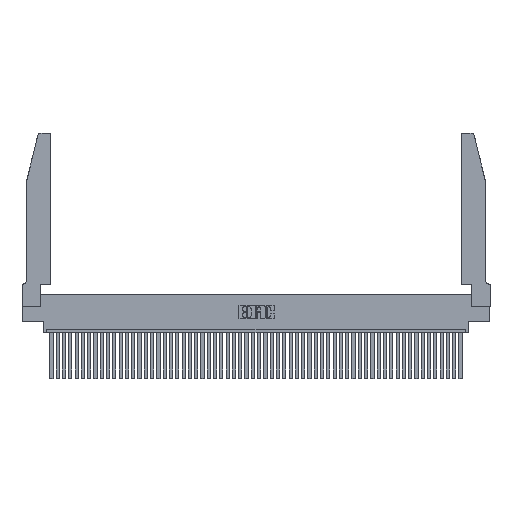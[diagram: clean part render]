
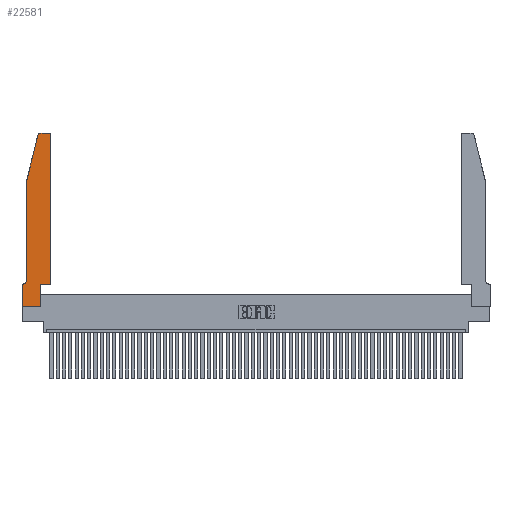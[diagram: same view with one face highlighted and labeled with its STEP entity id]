
A CAD part, top view. The second image highlights one B-rep face of the part: STEP entity #22581.
In plain terms, the highlighted planar face has unit normal (0, 0, 1).
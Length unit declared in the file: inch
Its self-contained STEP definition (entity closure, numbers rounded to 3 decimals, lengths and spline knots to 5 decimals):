
#289 = EDGE_CURVE ( 'NONE', #35568, #41114, #4312, .T. ) ;
#635 = ORIENTED_EDGE ( 'NONE', *, *, #289, .T. ) ;
#738 = AXIS2_PLACEMENT_3D ( 'NONE', #3399, #35102, #23356 ) ;
#847 = VERTEX_POINT ( 'NONE', #31609 ) ;
#1453 = VECTOR ( 'NONE', #14521, 39.37008 ) ;
#2069 = DIRECTION ( 'NONE',  ( -0.239, -0.971, 0. ) ) ;
#2330 = CARTESIAN_POINT ( 'NONE',  ( 0., 0., 0.37 ) ) ;
#2375 = LINE ( 'NONE', #38736, #33975 ) ;
#2720 = CARTESIAN_POINT ( 'NONE',  ( 0.4505, 0.35, 0.37 ) ) ;
#2827 = ORIENTED_EDGE ( 'NONE', *, *, #40851, .T. ) ;
#3399 = CARTESIAN_POINT ( 'NONE',  ( 0.0055, 0.42, 0.37 ) ) ;
#3774 = VERTEX_POINT ( 'NONE', #2330 ) ;
#4251 = CARTESIAN_POINT ( 'NONE',  ( 0.0055, 0.35, 0.37 ) ) ;
#4275 = DIRECTION ( 'NONE',  ( -1., 0., 0. ) ) ;
#4312 = LINE ( 'NONE', #29773, #12376 ) ;
#4354 = CARTESIAN_POINT ( 'NONE',  ( 0.0755, 2., 0.37 ) ) ;
#6153 = DIRECTION ( 'NONE',  ( 0., -1., 0. ) ) ;
#6306 = CARTESIAN_POINT ( 'NONE',  ( 0.0755, 0.35, 0.37 ) ) ;
#6374 = DIRECTION ( 'NONE',  ( 1., 0., 0. ) ) ;
#6639 = DIRECTION ( 'NONE',  ( 0., 0., 1. ) ) ;
#7251 = DIRECTION ( 'NONE',  ( 1., 0., 0. ) ) ;
#8568 = ORIENTED_EDGE ( 'NONE', *, *, #30644, .T. ) ;
#9077 = LINE ( 'NONE', #23287, #9700 ) ;
#9700 = VECTOR ( 'NONE', #30693, 39.37008 ) ;
#9938 = CARTESIAN_POINT ( 'NONE',  ( 0.4505, 0.35, 0.37 ) ) ;
#10612 = PLANE ( 'NONE',  #38066 ) ;
#11401 = VERTEX_POINT ( 'NONE', #32820 ) ;
#11506 = EDGE_CURVE ( 'NONE', #3774, #25291, #43487, .T. ) ;
#12145 = VERTEX_POINT ( 'NONE', #9938 ) ;
#12376 = VECTOR ( 'NONE', #2069, 39.37008 ) ;
#12937 = AXIS2_PLACEMENT_3D ( 'NONE', #29417, #33943, #45576 ) ;
#13068 = EDGE_CURVE ( 'NONE', #48024, #13459, #20467, .T. ) ;
#13267 = CARTESIAN_POINT ( 'NONE',  ( 0.284, 2.75, 0.37 ) ) ;
#13459 = VERTEX_POINT ( 'NONE', #18127 ) ;
#14521 = DIRECTION ( 'NONE',  ( 0., 1., 0. ) ) ;
#14974 = CARTESIAN_POINT ( 'NONE',  ( 0., 0., 0.37 ) ) ;
#15345 = CARTESIAN_POINT ( 'NONE',  ( 0.2865, 0., 0.37 ) ) ;
#15667 = EDGE_CURVE ( 'NONE', #15916, #847, #38754, .T. ) ;
#15916 = VERTEX_POINT ( 'NONE', #4251 ) ;
#16276 = CIRCLE ( 'NONE', #738, 0.07 ) ;
#17100 = ORIENTED_EDGE ( 'NONE', *, *, #45932, .T. ) ;
#17603 = DIRECTION ( 'NONE',  ( 0., -1., 0. ) ) ;
#18127 = CARTESIAN_POINT ( 'NONE',  ( 0.4205, 2.75, 0.37 ) ) ;
#18421 = CARTESIAN_POINT ( 'NONE',  ( 0.4505, 2.72, 0.37 ) ) ;
#18879 = DIRECTION ( 'NONE',  ( 1., 0., 0. ) ) ;
#19438 = EDGE_LOOP ( 'NONE', ( #8568, #28734, #635, #33978, #40231, #34110, #19447, #33053, #17100, #2827, #30735, #37930 ) ) ;
#19447 = ORIENTED_EDGE ( 'NONE', *, *, #36415, .T. ) ;
#19859 = LINE ( 'NONE', #45656, #29134 ) ;
#20467 = CIRCLE ( 'NONE', #12937, 0.03 ) ;
#20698 = VERTEX_POINT ( 'NONE', #26058 ) ;
#20799 = VECTOR ( 'NONE', #17603, 39.37008 ) ;
#21427 = CARTESIAN_POINT ( 'NONE',  ( 0.25487, 2.72718, 0.37 ) ) ;
#22581 = ADVANCED_FACE ( 'NONE', ( #44597 ), #10612, .T. ) ;
#22766 = LINE ( 'NONE', #28332, #20799 ) ;
#23287 = CARTESIAN_POINT ( 'NONE',  ( 0.2605, 2.75, 0.37 ) ) ;
#23356 = DIRECTION ( 'NONE',  ( -1., 0., 0. ) ) ;
#24533 = VECTOR ( 'NONE', #4275, 39.37008 ) ;
#25291 = VERTEX_POINT ( 'NONE', #15345 ) ;
#26058 = CARTESIAN_POINT ( 'NONE',  ( 0.0755, 0.42, 0.37 ) ) ;
#26113 = EDGE_CURVE ( 'NONE', #41114, #20698, #22766, .T. ) ;
#27490 = EDGE_CURVE ( 'NONE', #20698, #15916, #16276, .T. ) ;
#27770 = CIRCLE ( 'NONE', #35228, 0.03 ) ;
#28332 = CARTESIAN_POINT ( 'NONE',  ( 0.0755, 2., 0.37 ) ) ;
#28734 = ORIENTED_EDGE ( 'NONE', *, *, #37748, .T. ) ;
#29134 = VECTOR ( 'NONE', #6153, 39.37008 ) ;
#29417 = CARTESIAN_POINT ( 'NONE',  ( 0.4205, 2.72, 0.37 ) ) ;
#29773 = CARTESIAN_POINT ( 'NONE',  ( 0.0755, 2., 0.37 ) ) ;
#30080 = LINE ( 'NONE', #34478, #1453 ) ;
#30644 = EDGE_CURVE ( 'NONE', #13459, #35480, #9077, .T. ) ;
#30693 = DIRECTION ( 'NONE',  ( -1., 0., 0. ) ) ;
#30735 = ORIENTED_EDGE ( 'NONE', *, *, #42153, .T. ) ;
#31609 = CARTESIAN_POINT ( 'NONE',  ( 0., 0.35, 0.37 ) ) ;
#32820 = CARTESIAN_POINT ( 'NONE',  ( 0.2865, 0.35, 0.37 ) ) ;
#33053 = ORIENTED_EDGE ( 'NONE', *, *, #11506, .T. ) ;
#33278 = DIRECTION ( 'NONE',  ( 1., 0., 0. ) ) ;
#33943 = DIRECTION ( 'NONE',  ( 0., 0., 1. ) ) ;
#33975 = VECTOR ( 'NONE', #42666, 39.37008 ) ;
#33978 = ORIENTED_EDGE ( 'NONE', *, *, #26113, .T. ) ;
#34007 = CARTESIAN_POINT ( 'NONE',  ( 0.284, 2.72, 0.37 ) ) ;
#34110 = ORIENTED_EDGE ( 'NONE', *, *, #15667, .T. ) ;
#34478 = CARTESIAN_POINT ( 'NONE',  ( 0.4505, 0.35, 0.37 ) ) ;
#35102 = DIRECTION ( 'NONE',  ( 0., 0., -1. ) ) ;
#35228 = AXIS2_PLACEMENT_3D ( 'NONE', #34007, #49109, #33278 ) ;
#35480 = VERTEX_POINT ( 'NONE', #13267 ) ;
#35568 = VERTEX_POINT ( 'NONE', #21427 ) ;
#36415 = EDGE_CURVE ( 'NONE', #847, #3774, #19859, .T. ) ;
#37748 = EDGE_CURVE ( 'NONE', #35480, #35568, #27770, .T. ) ;
#37930 = ORIENTED_EDGE ( 'NONE', *, *, #13068, .T. ) ;
#38066 = AXIS2_PLACEMENT_3D ( 'NONE', #38908, #6639, #18879 ) ;
#38736 = CARTESIAN_POINT ( 'NONE',  ( 0.2865, 0.35, 0.37 ) ) ;
#38754 = LINE ( 'NONE', #6306, #24533 ) ;
#38908 = CARTESIAN_POINT ( 'NONE',  ( 0., 0.35, 0.37 ) ) ;
#40231 = ORIENTED_EDGE ( 'NONE', *, *, #27490, .T. ) ;
#40851 = EDGE_CURVE ( 'NONE', #11401, #12145, #48385, .T. ) ;
#41114 = VERTEX_POINT ( 'NONE', #4354 ) ;
#42153 = EDGE_CURVE ( 'NONE', #12145, #48024, #30080, .T. ) ;
#42666 = DIRECTION ( 'NONE',  ( 0., 1., 0. ) ) ;
#43487 = LINE ( 'NONE', #14974, #44677 ) ;
#44597 = FACE_OUTER_BOUND ( 'NONE', #19438, .T. ) ;
#44677 = VECTOR ( 'NONE', #7251, 39.37008 ) ;
#45289 = VECTOR ( 'NONE', #6374, 39.37008 ) ;
#45576 = DIRECTION ( 'NONE',  ( 1., 0., 0. ) ) ;
#45656 = CARTESIAN_POINT ( 'NONE',  ( 0., 0., 0.37 ) ) ;
#45932 = EDGE_CURVE ( 'NONE', #25291, #11401, #2375, .T. ) ;
#48024 = VERTEX_POINT ( 'NONE', #18421 ) ;
#48385 = LINE ( 'NONE', #2720, #45289 ) ;
#49109 = DIRECTION ( 'NONE',  ( 0., 0., 1. ) ) ;
